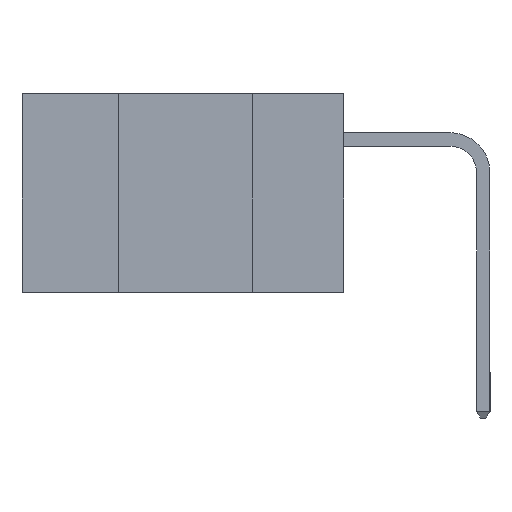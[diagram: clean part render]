
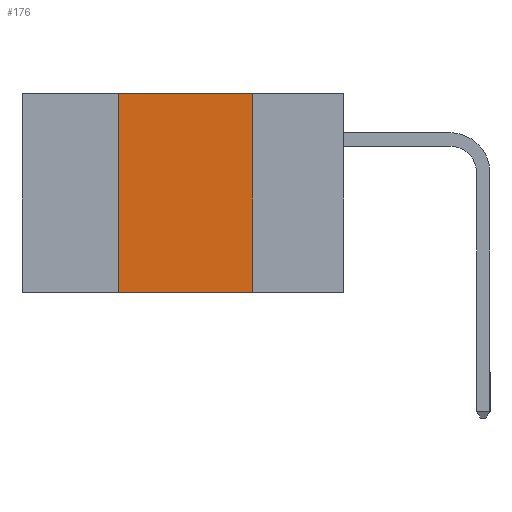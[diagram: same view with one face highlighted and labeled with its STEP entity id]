
A CAD part, left-side view. The second image highlights one B-rep face of the part: STEP entity #176.
In plain terms, the highlighted planar face has unit normal (-1, 0, 0).
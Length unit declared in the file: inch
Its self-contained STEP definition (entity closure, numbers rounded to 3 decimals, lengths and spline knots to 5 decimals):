
#142 = DIRECTION ( 'NONE',  ( 0., -1., 0. ) ) ;
#160 = EDGE_CURVE ( 'NONE', #6951, #1748, #5060, .T. ) ;
#176 = ADVANCED_FACE ( 'NONE', ( #8506 ), #7970, .F. ) ;
#200 = DIRECTION ( 'NONE',  ( 0., 0., 1. ) ) ;
#400 = CARTESIAN_POINT ( 'NONE',  ( 0., 0.17, -0.37 ) ) ;
#454 = LINE ( 'NONE', #400, #2191 ) ;
#1230 = ORIENTED_EDGE ( 'NONE', *, *, #7567, .F. ) ;
#1736 = CARTESIAN_POINT ( 'NONE',  ( 0., 0.17, 0. ) ) ;
#1748 = VERTEX_POINT ( 'NONE', #8378 ) ;
#2191 = VECTOR ( 'NONE', #3269, 39.37008 ) ;
#2286 = LINE ( 'NONE', #5079, #3650 ) ;
#2316 = DIRECTION ( 'NONE',  ( 0., 0., -1. ) ) ;
#3052 = CARTESIAN_POINT ( 'NONE',  ( 0., 0.6, -0.37 ) ) ;
#3269 = DIRECTION ( 'NONE',  ( 0., 0., -1. ) ) ;
#3650 = VECTOR ( 'NONE', #200, 39.37008 ) ;
#3767 = CARTESIAN_POINT ( 'NONE',  ( 0., 0.6, 0. ) ) ;
#4326 = VERTEX_POINT ( 'NONE', #1736 ) ;
#4550 = EDGE_LOOP ( 'NONE', ( #7998, #1230, #5269, #7073 ) ) ;
#4570 = VERTEX_POINT ( 'NONE', #5023 ) ;
#4696 = AXIS2_PLACEMENT_3D ( 'NONE', #3767, #7798, #2316 ) ;
#5023 = CARTESIAN_POINT ( 'NONE',  ( 0., 0.42, 0. ) ) ;
#5025 = LINE ( 'NONE', #6988, #7760 ) ;
#5060 = LINE ( 'NONE', #3052, #5996 ) ;
#5079 = CARTESIAN_POINT ( 'NONE',  ( 0., 0.42, -0.37 ) ) ;
#5269 = ORIENTED_EDGE ( 'NONE', *, *, #5547, .F. ) ;
#5274 = EDGE_CURVE ( 'NONE', #4326, #1748, #454, .T. ) ;
#5547 = EDGE_CURVE ( 'NONE', #6951, #4570, #2286, .T. ) ;
#5648 = DIRECTION ( 'NONE',  ( 0., -1., 0. ) ) ;
#5996 = VECTOR ( 'NONE', #142, 39.37008 ) ;
#6951 = VERTEX_POINT ( 'NONE', #8623 ) ;
#6988 = CARTESIAN_POINT ( 'NONE',  ( 0., 0.6, 0. ) ) ;
#7073 = ORIENTED_EDGE ( 'NONE', *, *, #160, .T. ) ;
#7567 = EDGE_CURVE ( 'NONE', #4570, #4326, #5025, .T. ) ;
#7760 = VECTOR ( 'NONE', #5648, 39.37008 ) ;
#7798 = DIRECTION ( 'NONE',  ( 1., 0., 0. ) ) ;
#7970 = PLANE ( 'NONE',  #4696 ) ;
#7998 = ORIENTED_EDGE ( 'NONE', *, *, #5274, .F. ) ;
#8378 = CARTESIAN_POINT ( 'NONE',  ( 0., 0.17, -0.37 ) ) ;
#8506 = FACE_OUTER_BOUND ( 'NONE', #4550, .T. ) ;
#8623 = CARTESIAN_POINT ( 'NONE',  ( 0., 0.42, -0.37 ) ) ;
